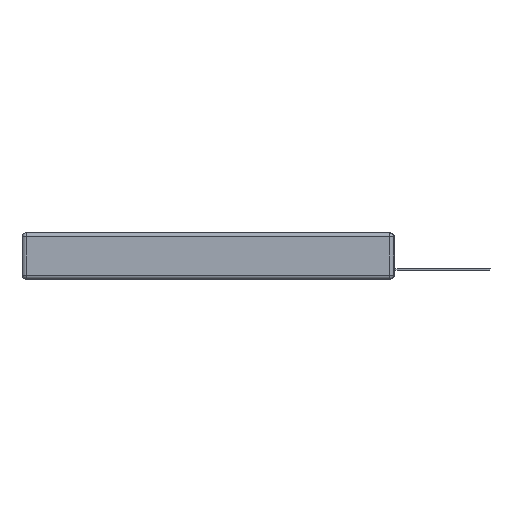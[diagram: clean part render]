
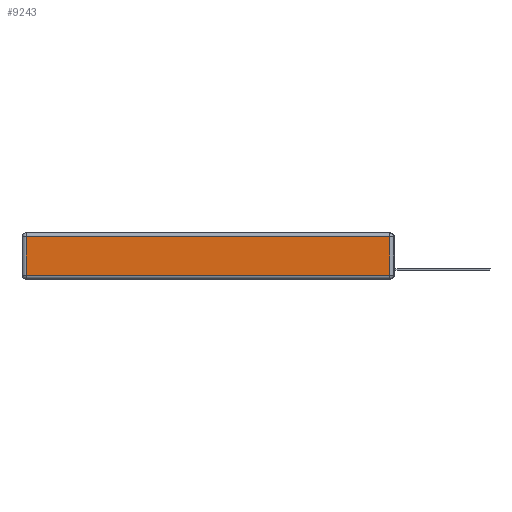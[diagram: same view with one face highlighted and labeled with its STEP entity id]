
A CAD part, left-side view. The second image highlights one B-rep face of the part: STEP entity #9243.
In plain terms, the highlighted planar face has unit normal (-1, 0, 0).
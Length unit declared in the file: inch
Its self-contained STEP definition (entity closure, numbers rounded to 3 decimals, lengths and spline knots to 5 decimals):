
#22 = DIRECTION ( 'NONE',  ( 0., 1., 0. ) ) ;
#316 = DIRECTION ( 'NONE',  ( 0., -1., 0. ) ) ;
#592 = VERTEX_POINT ( 'NONE', #12240 ) ;
#1407 = VECTOR ( 'NONE', #20667, 39.37008 ) ;
#1532 = VECTOR ( 'NONE', #22, 39.37008 ) ;
#1548 = CARTESIAN_POINT ( 'NONE',  ( 0., 2.75, -0.03 ) ) ;
#1756 = EDGE_LOOP ( 'NONE', ( #4254, #16615, #4702, #11037 ) ) ;
#1846 = CARTESIAN_POINT ( 'NONE',  ( 0., 2.72, -0.03 ) ) ;
#2140 = VERTEX_POINT ( 'NONE', #5575 ) ;
#4088 = LINE ( 'NONE', #15761, #9864 ) ;
#4254 = ORIENTED_EDGE ( 'NONE', *, *, #16042, .T. ) ;
#4702 = ORIENTED_EDGE ( 'NONE', *, *, #23039, .T. ) ;
#5575 = CARTESIAN_POINT ( 'NONE',  ( 0., 0.03, -0.03 ) ) ;
#6080 = CARTESIAN_POINT ( 'NONE',  ( 0., 0., -0.343 ) ) ;
#7835 = PLANE ( 'NONE',  #21539 ) ;
#8209 = DIRECTION ( 'NONE',  ( 0., 0., 1. ) ) ;
#8407 = CARTESIAN_POINT ( 'NONE',  ( 0., 2.72, -0.313 ) ) ;
#8665 = VERTEX_POINT ( 'NONE', #8407 ) ;
#9149 = EDGE_CURVE ( 'NONE', #592, #2140, #22752, .T. ) ;
#9243 = ADVANCED_FACE ( 'NONE', ( #17488 ), #7835, .T. ) ;
#9268 = CARTESIAN_POINT ( 'NONE',  ( 0., 2.72, -0.343 ) ) ;
#9349 = CARTESIAN_POINT ( 'NONE',  ( 0., 0.03, -0.343 ) ) ;
#9864 = VECTOR ( 'NONE', #316, 39.37008 ) ;
#11037 = ORIENTED_EDGE ( 'NONE', *, *, #18783, .T. ) ;
#12240 = CARTESIAN_POINT ( 'NONE',  ( 0., 0.03, -0.313 ) ) ;
#15761 = CARTESIAN_POINT ( 'NONE',  ( 0., 0., -0.313 ) ) ;
#16042 = EDGE_CURVE ( 'NONE', #8665, #592, #4088, .T. ) ;
#16534 = LINE ( 'NONE', #9268, #1407 ) ;
#16615 = ORIENTED_EDGE ( 'NONE', *, *, #9149, .T. ) ;
#17222 = LINE ( 'NONE', #1548, #1532 ) ;
#17488 = FACE_OUTER_BOUND ( 'NONE', #1756, .T. ) ;
#18783 = EDGE_CURVE ( 'NONE', #18895, #8665, #16534, .T. ) ;
#18895 = VERTEX_POINT ( 'NONE', #1846 ) ;
#20667 = DIRECTION ( 'NONE',  ( 0., 0., -1. ) ) ;
#20749 = VECTOR ( 'NONE', #20755, 39.37008 ) ;
#20755 = DIRECTION ( 'NONE',  ( 0., 0., 1. ) ) ;
#21123 = DIRECTION ( 'NONE',  ( -1., 0., 0. ) ) ;
#21539 = AXIS2_PLACEMENT_3D ( 'NONE', #6080, #21123, #8209 ) ;
#22752 = LINE ( 'NONE', #9349, #20749 ) ;
#23039 = EDGE_CURVE ( 'NONE', #2140, #18895, #17222, .T. ) ;
